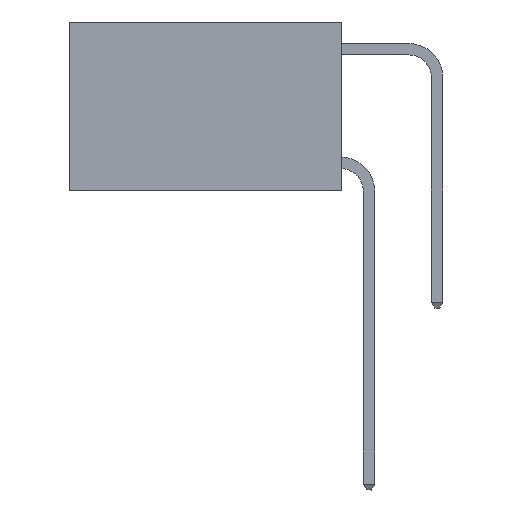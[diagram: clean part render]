
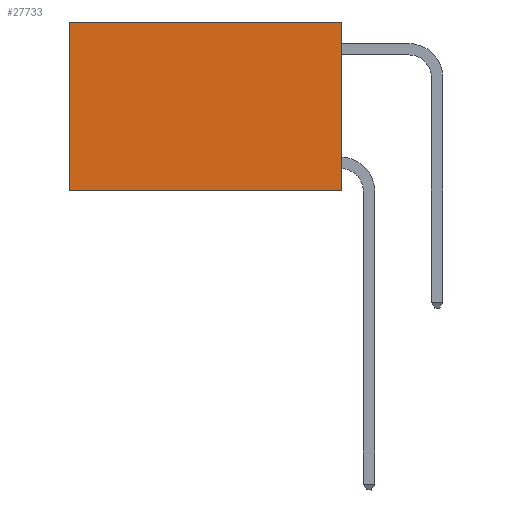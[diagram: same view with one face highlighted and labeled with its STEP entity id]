
A CAD part, left-side view. The second image highlights one B-rep face of the part: STEP entity #27733.
In plain terms, the highlighted planar face has unit normal (-1, 0, 0).
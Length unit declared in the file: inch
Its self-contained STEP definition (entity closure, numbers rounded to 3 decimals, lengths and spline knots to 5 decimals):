
#1742 = CARTESIAN_POINT ( 'NONE',  ( 0.2625, 0.6, 0. ) ) ;
#2158 = LINE ( 'NONE', #17140, #30822 ) ;
#3777 = CARTESIAN_POINT ( 'NONE',  ( 0.2625, 0., 0. ) ) ;
#3831 = ORIENTED_EDGE ( 'NONE', *, *, #16328, .T. ) ;
#4017 = VECTOR ( 'NONE', #15669, 39.37008 ) ;
#6719 = DIRECTION ( 'NONE',  ( 0., 0., -1. ) ) ;
#7044 = VERTEX_POINT ( 'NONE', #20665 ) ;
#8283 = CARTESIAN_POINT ( 'NONE',  ( 0.2625, 0., 0. ) ) ;
#8667 = CARTESIAN_POINT ( 'NONE',  ( 0.2625, 0., 0. ) ) ;
#9292 = DIRECTION ( 'NONE',  ( 1., 0., 0. ) ) ;
#9325 = CARTESIAN_POINT ( 'NONE',  ( 0.2625, 0., -0.37 ) ) ;
#11005 = DIRECTION ( 'NONE',  ( 0., 0., -1. ) ) ;
#11238 = CARTESIAN_POINT ( 'NONE',  ( 0.2625, 0.6, 0. ) ) ;
#13256 = DIRECTION ( 'NONE',  ( 0., 0., -1. ) ) ;
#13545 = CARTESIAN_POINT ( 'NONE',  ( 0.2625, 0., -0.37 ) ) ;
#13556 = EDGE_CURVE ( 'NONE', #27936, #7044, #15564, .T. ) ;
#13685 = VECTOR ( 'NONE', #11005, 39.37008 ) ;
#14246 = VERTEX_POINT ( 'NONE', #8667 ) ;
#15141 = EDGE_LOOP ( 'NONE', ( #3831, #29050, #15588, #20278 ) ) ;
#15564 = LINE ( 'NONE', #13545, #4017 ) ;
#15588 = ORIENTED_EDGE ( 'NONE', *, *, #18427, .F. ) ;
#15669 = DIRECTION ( 'NONE',  ( 0., 1., 0. ) ) ;
#16328 = EDGE_CURVE ( 'NONE', #20561, #7044, #20252, .T. ) ;
#17140 = CARTESIAN_POINT ( 'NONE',  ( 0.2625, 0., 0. ) ) ;
#18427 = EDGE_CURVE ( 'NONE', #14246, #27936, #30996, .T. ) ;
#20252 = LINE ( 'NONE', #11238, #13685 ) ;
#20278 = ORIENTED_EDGE ( 'NONE', *, *, #26903, .T. ) ;
#20561 = VERTEX_POINT ( 'NONE', #1742 ) ;
#20665 = CARTESIAN_POINT ( 'NONE',  ( 0.2625, 0.6, -0.37 ) ) ;
#20838 = DIRECTION ( 'NONE',  ( 0., 1., 0. ) ) ;
#24130 = FACE_OUTER_BOUND ( 'NONE', #15141, .T. ) ;
#26903 = EDGE_CURVE ( 'NONE', #14246, #20561, #2158, .T. ) ;
#27499 = VECTOR ( 'NONE', #13256, 39.37008 ) ;
#27733 = ADVANCED_FACE ( 'NONE', ( #24130 ), #28233, .F. ) ;
#27936 = VERTEX_POINT ( 'NONE', #9325 ) ;
#28233 = PLANE ( 'NONE',  #28858 ) ;
#28858 = AXIS2_PLACEMENT_3D ( 'NONE', #3777, #9292, #6719 ) ;
#29050 = ORIENTED_EDGE ( 'NONE', *, *, #13556, .F. ) ;
#30822 = VECTOR ( 'NONE', #20838, 39.37008 ) ;
#30996 = LINE ( 'NONE', #8283, #27499 ) ;
